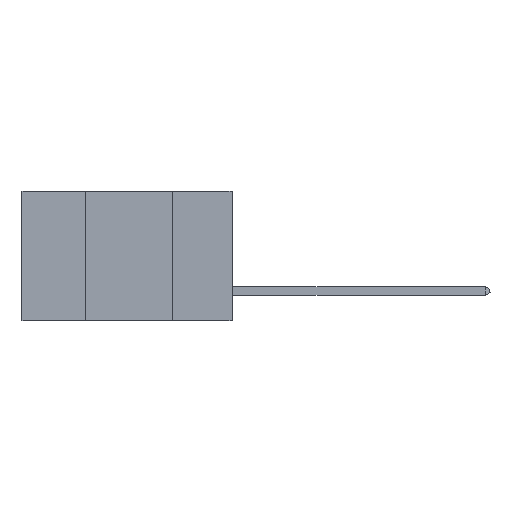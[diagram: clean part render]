
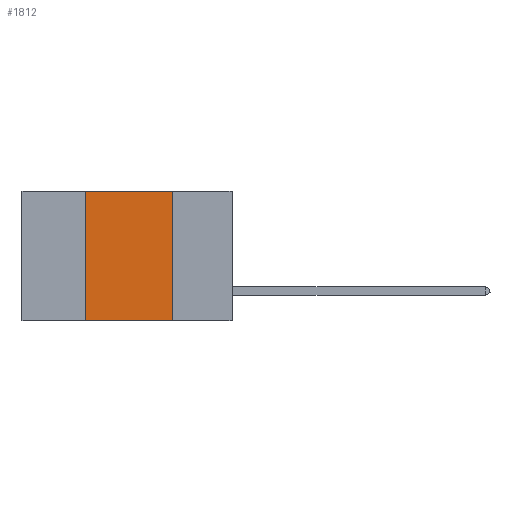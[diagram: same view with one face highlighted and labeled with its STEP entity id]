
A CAD part, left-side view. The second image highlights one B-rep face of the part: STEP entity #1812.
In plain terms, the highlighted planar face has unit normal (-1, 0, 0).
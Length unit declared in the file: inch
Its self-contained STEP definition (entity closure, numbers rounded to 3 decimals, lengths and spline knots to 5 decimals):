
#258 = EDGE_CURVE ( 'NONE', #9512, #13584, #10122, .T. ) ;
#349 = VERTEX_POINT ( 'NONE', #13875 ) ;
#1375 = CARTESIAN_POINT ( 'NONE',  ( 0., 0.17, -0.37 ) ) ;
#1395 = ORIENTED_EDGE ( 'NONE', *, *, #7217, .F. ) ;
#1434 = FACE_OUTER_BOUND ( 'NONE', #5920, .T. ) ;
#1812 = ADVANCED_FACE ( 'NONE', ( #1434 ), #11837, .F. ) ;
#2165 = CARTESIAN_POINT ( 'NONE',  ( 0., 0.42, 0. ) ) ;
#3632 = EDGE_CURVE ( 'NONE', #349, #13584, #12181, .T. ) ;
#3699 = EDGE_CURVE ( 'NONE', #7296, #9512, #10809, .T. ) ;
#3710 = DIRECTION ( 'NONE',  ( 0., 0., -1. ) ) ;
#4117 = DIRECTION ( 'NONE',  ( 0., -1., 0. ) ) ;
#4200 = DIRECTION ( 'NONE',  ( 1., 0., 0. ) ) ;
#4300 = CARTESIAN_POINT ( 'NONE',  ( 0., 0.6, 0. ) ) ;
#4642 = LINE ( 'NONE', #13555, #5067 ) ;
#4759 = CARTESIAN_POINT ( 'NONE',  ( 0., 0.17, 0. ) ) ;
#4801 = ORIENTED_EDGE ( 'NONE', *, *, #258, .F. ) ;
#5067 = VECTOR ( 'NONE', #6047, 39.37008 ) ;
#5310 = CARTESIAN_POINT ( 'NONE',  ( 0., 0.6, -0.37 ) ) ;
#5920 = EDGE_LOOP ( 'NONE', ( #4801, #6748, #1395, #14095 ) ) ;
#6047 = DIRECTION ( 'NONE',  ( 0., 0., 1. ) ) ;
#6625 = CARTESIAN_POINT ( 'NONE',  ( 0., 0.6, 0. ) ) ;
#6748 = ORIENTED_EDGE ( 'NONE', *, *, #3699, .F. ) ;
#7217 = EDGE_CURVE ( 'NONE', #349, #7296, #4642, .T. ) ;
#7296 = VERTEX_POINT ( 'NONE', #2165 ) ;
#8624 = CARTESIAN_POINT ( 'NONE',  ( 0., 0.17, 0. ) ) ;
#9512 = VERTEX_POINT ( 'NONE', #8624 ) ;
#10122 = LINE ( 'NONE', #4759, #12506 ) ;
#10809 = LINE ( 'NONE', #6625, #13179 ) ;
#10893 = AXIS2_PLACEMENT_3D ( 'NONE', #4300, #4200, #14320 ) ;
#11837 = PLANE ( 'NONE',  #10893 ) ;
#12181 = LINE ( 'NONE', #5310, #14369 ) ;
#12506 = VECTOR ( 'NONE', #3710, 39.37008 ) ;
#13179 = VECTOR ( 'NONE', #4117, 39.37008 ) ;
#13555 = CARTESIAN_POINT ( 'NONE',  ( 0., 0.42, 0. ) ) ;
#13584 = VERTEX_POINT ( 'NONE', #1375 ) ;
#13875 = CARTESIAN_POINT ( 'NONE',  ( 0., 0.42, -0.37 ) ) ;
#14095 = ORIENTED_EDGE ( 'NONE', *, *, #3632, .T. ) ;
#14141 = DIRECTION ( 'NONE',  ( 0., -1., 0. ) ) ;
#14320 = DIRECTION ( 'NONE',  ( 0., 0., -1. ) ) ;
#14369 = VECTOR ( 'NONE', #14141, 39.37008 ) ;
